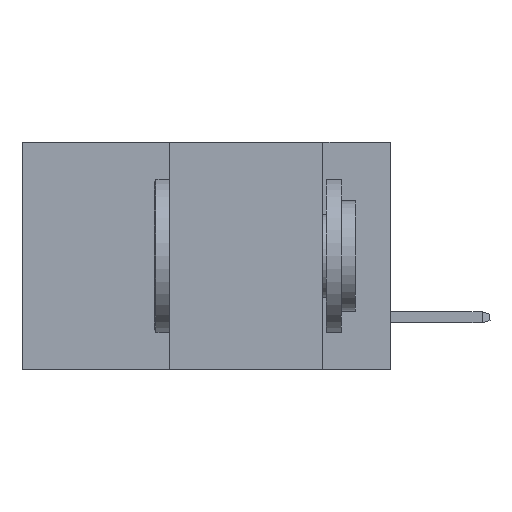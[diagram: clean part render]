
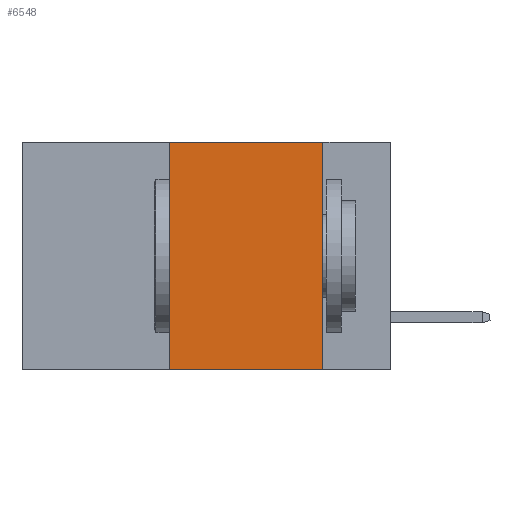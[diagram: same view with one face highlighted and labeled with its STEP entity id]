
A CAD part, left-side view. The second image highlights one B-rep face of the part: STEP entity #6548.
In plain terms, the highlighted planar face has unit normal (-1, 0, 0).
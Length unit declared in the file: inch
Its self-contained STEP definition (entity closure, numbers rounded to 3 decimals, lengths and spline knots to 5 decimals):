
#506 = CARTESIAN_POINT ( 'NONE',  ( 0., 0.36, 0. ) ) ;
#1048 = EDGE_LOOP ( 'NONE', ( #11614, #7931, #7356, #2122 ) ) ;
#1176 = EDGE_CURVE ( 'NONE', #13758, #6921, #13222, .T. ) ;
#1423 = VECTOR ( 'NONE', #6372, 39.37008 ) ;
#1445 = FACE_OUTER_BOUND ( 'NONE', #1048, .T. ) ;
#2122 = ORIENTED_EDGE ( 'NONE', *, *, #12519, .T. ) ;
#2193 = EDGE_CURVE ( 'NONE', #12468, #13758, #9939, .T. ) ;
#2580 = DIRECTION ( 'NONE',  ( 0., 0., -1. ) ) ;
#3270 = VECTOR ( 'NONE', #2580, 39.37008 ) ;
#3393 = PLANE ( 'NONE',  #14610 ) ;
#3434 = DIRECTION ( 'NONE',  ( 0., -1., 0. ) ) ;
#3765 = CARTESIAN_POINT ( 'NONE',  ( 0., 0.11, -0.37 ) ) ;
#3831 = LINE ( 'NONE', #6060, #3270 ) ;
#4438 = LINE ( 'NONE', #8272, #13815 ) ;
#4607 = CARTESIAN_POINT ( 'NONE',  ( 0., 0.6, 0. ) ) ;
#4781 = CARTESIAN_POINT ( 'NONE',  ( 0., 0.36, -0.37 ) ) ;
#6060 = CARTESIAN_POINT ( 'NONE',  ( 0., 0.11, 0. ) ) ;
#6372 = DIRECTION ( 'NONE',  ( 0., -1., 0. ) ) ;
#6548 = ADVANCED_FACE ( 'NONE', ( #1445 ), #3393, .F. ) ;
#6921 = VERTEX_POINT ( 'NONE', #8549 ) ;
#7251 = VECTOR ( 'NONE', #7820, 39.37008 ) ;
#7356 = ORIENTED_EDGE ( 'NONE', *, *, #2193, .F. ) ;
#7820 = DIRECTION ( 'NONE',  ( 0., 0., 1. ) ) ;
#7931 = ORIENTED_EDGE ( 'NONE', *, *, #1176, .F. ) ;
#8123 = DIRECTION ( 'NONE',  ( 1., 0., 0. ) ) ;
#8212 = EDGE_CURVE ( 'NONE', #6921, #15147, #3831, .T. ) ;
#8272 = CARTESIAN_POINT ( 'NONE',  ( 0., 0.6, -0.37 ) ) ;
#8549 = CARTESIAN_POINT ( 'NONE',  ( 0., 0.11, 0. ) ) ;
#9306 = CARTESIAN_POINT ( 'NONE',  ( 0., 0.36, 0. ) ) ;
#9939 = LINE ( 'NONE', #506, #7251 ) ;
#11614 = ORIENTED_EDGE ( 'NONE', *, *, #8212, .F. ) ;
#12468 = VERTEX_POINT ( 'NONE', #4781 ) ;
#12519 = EDGE_CURVE ( 'NONE', #12468, #15147, #4438, .T. ) ;
#12999 = DIRECTION ( 'NONE',  ( 0., 0., -1. ) ) ;
#13222 = LINE ( 'NONE', #13772, #1423 ) ;
#13758 = VERTEX_POINT ( 'NONE', #9306 ) ;
#13772 = CARTESIAN_POINT ( 'NONE',  ( 0., 0.6, 0. ) ) ;
#13815 = VECTOR ( 'NONE', #3434, 39.37008 ) ;
#14610 = AXIS2_PLACEMENT_3D ( 'NONE', #4607, #8123, #12999 ) ;
#15147 = VERTEX_POINT ( 'NONE', #3765 ) ;
